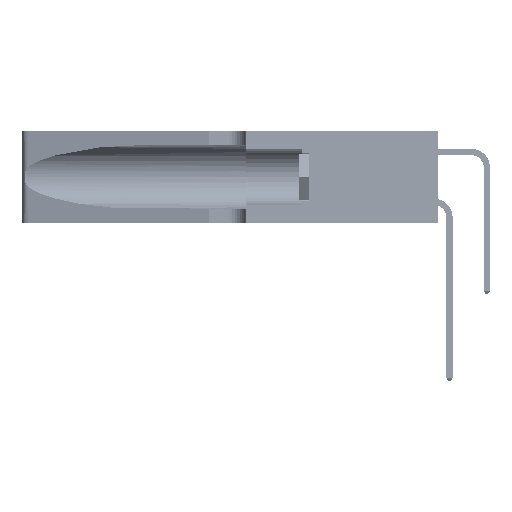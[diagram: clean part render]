
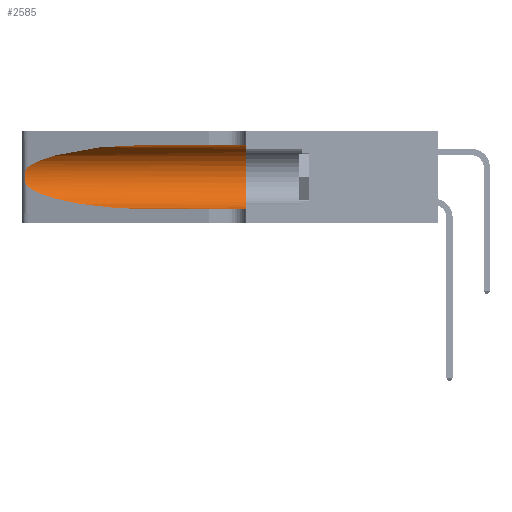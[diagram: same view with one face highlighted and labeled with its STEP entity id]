
A CAD part, left-side view. The second image highlights one B-rep face of the part: STEP entity #2585.
In plain terms, the highlighted cylindrical face has radius 3.308 mm (diameter 6.617 mm), a partial arc.
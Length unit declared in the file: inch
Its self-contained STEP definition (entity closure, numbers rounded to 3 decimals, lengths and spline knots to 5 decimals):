
#133 = LINE ( 'NONE', #42479, #29803 ) ;
#441 = CARTESIAN_POINT ( 'NONE',  ( 0.18966, 0.96281, 0.05475 ) ) ;
#765 = CARTESIAN_POINT ( 'NONE',  ( 0.25789, 1.23486, 0.15765 ) ) ;
#1041 = VERTEX_POINT ( 'NONE', #31571 ) ;
#2025 = VERTEX_POINT ( 'NONE', #5735 ) ;
#2585 = ADVANCED_FACE ( 'NONE', ( #38193 ), #37024, .F. ) ;
#3441 =( BOUNDED_CURVE ( )  B_SPLINE_CURVE ( 3, ( #19033, #22748, #441, #26458 ),
 .UNSPECIFIED., .F., .T. ) 
 B_SPLINE_CURVE_WITH_KNOTS ( ( 4, 4 ),
 ( 3.44316, 4.71239 ),
 .UNSPECIFIED. ) 
 CURVE ( )  GEOMETRIC_REPRESENTATION_ITEM ( )  RATIONAL_B_SPLINE_CURVE ( ( 1., 0.87, 0.87, 1. ) ) 
 REPRESENTATION_ITEM ( '' )  );
#4547 = CARTESIAN_POINT ( 'NONE',  ( 0.25555, 1.22993, 0.14849 ) ) ;
#4876 = ORIENTED_EDGE ( 'NONE', *, *, #35650, .T. ) ;
#5464 = CARTESIAN_POINT ( 'NONE',  ( 0.1305, 0.35, 0.185 ) ) ;
#5735 = CARTESIAN_POINT ( 'NONE',  ( 0.1305, 0.72297, 0.31525 ) ) ;
#5817 = CARTESIAN_POINT ( 'NONE',  ( 0.1305, 0.72297, 0.31525 ) ) ;
#6913 = ORIENTED_EDGE ( 'NONE', *, *, #13393, .F. ) ;
#7002 = CIRCLE ( 'NONE', #17440, 0.13025 ) ;
#8026 = EDGE_CURVE ( 'NONE', #2025, #17849, #10770, .T. ) ;
#8785 = CARTESIAN_POINT ( 'NONE',  ( 0.1305, 1.61858, 0.185 ) ) ;
#9190 = DIRECTION ( 'NONE',  ( 0., 0., 1. ) ) ;
#9556 = CARTESIAN_POINT ( 'NONE',  ( 0.2373, 1.15595, 0.28018 ) ) ;
#9574 = VECTOR ( 'NONE', #47803, 39.37008 ) ;
#10770 = LINE ( 'NONE', #44153, #9574 ) ;
#11849 = CARTESIAN_POINT ( 'NONE',  ( 0.25787, 1.23484, 0.2124 ) ) ;
#13393 = EDGE_CURVE ( 'NONE', #17849, #45125, #7002, .T. ) ;
#15618 = CARTESIAN_POINT ( 'NONE',  ( 0.26018, 1.23835, 0.19895 ) ) ;
#16298 = DIRECTION ( 'NONE',  ( 0., -1., 0. ) ) ;
#16545 = VERTEX_POINT ( 'NONE', #37351 ) ;
#17440 = AXIS2_PLACEMENT_3D ( 'NONE', #5464, #31432, #9190 ) ;
#17849 = VERTEX_POINT ( 'NONE', #35710 ) ;
#19033 = CARTESIAN_POINT ( 'NONE',  ( 0.25487, 1.22718, 0.14631 ) ) ;
#19349 = CARTESIAN_POINT ( 'NONE',  ( 0.26075, 1.23896, 0.178 ) ) ;
#19716 = ORIENTED_EDGE ( 'NONE', *, *, #25425, .T. ) ;
#21882 = ORIENTED_EDGE ( 'NONE', *, *, #47232, .T. ) ;
#22748 = CARTESIAN_POINT ( 'NONE',  ( 0.2373, 1.15595, 0.08982 ) ) ;
#22784 = ORIENTED_EDGE ( 'NONE', *, *, #8026, .F. ) ;
#23077 = CARTESIAN_POINT ( 'NONE',  ( 0.25856, 1.23593, 0.16098 ) ) ;
#25425 = EDGE_CURVE ( 'NONE', #2025, #1041, #29337, .T. ) ;
#25695 = ORIENTED_EDGE ( 'NONE', *, *, #47913, .T. ) ;
#26458 = CARTESIAN_POINT ( 'NONE',  ( 0.1305, 0.72297, 0.05475 ) ) ;
#26766 = CARTESIAN_POINT ( 'NONE',  ( 0.25639, 1.23186, 0.15144 ) ) ;
#28071 = CARTESIAN_POINT ( 'NONE',  ( 0.18966, 0.96281, 0.31525 ) ) ;
#29337 =( BOUNDED_CURVE ( )  B_SPLINE_CURVE ( 3, ( #5817, #28071, #9556, #35576 ),
 .UNSPECIFIED., .F., .F. ) 
 B_SPLINE_CURVE_WITH_KNOTS ( ( 4, 4 ),
 ( 1.5708, 2.84003 ),
 .UNSPECIFIED. ) 
 CURVE ( )  GEOMETRIC_REPRESENTATION_ITEM ( )  RATIONAL_B_SPLINE_CURVE ( ( 1., 0.87, 0.87, 1. ) ) 
 REPRESENTATION_ITEM ( '' )  );
#29803 = VECTOR ( 'NONE', #31468, 39.37008 ) ;
#30338 = CARTESIAN_POINT ( 'NONE',  ( 0.25555, 1.22994, 0.2215 ) ) ;
#30515 = CARTESIAN_POINT ( 'NONE',  ( 0.25487, 1.22718, 0.14631 ) ) ;
#30672 = VERTEX_POINT ( 'NONE', #45387 ) ;
#31014 = DIRECTION ( 'NONE',  ( 0., 0., -1. ) ) ;
#31432 = DIRECTION ( 'NONE',  ( 0., 1., 0. ) ) ;
#31468 = DIRECTION ( 'NONE',  ( 0., -1., 0. ) ) ;
#31571 = CARTESIAN_POINT ( 'NONE',  ( 0.25487, 1.22718, 0.22369 ) ) ;
#32955 = CARTESIAN_POINT ( 'NONE',  ( 0.1305, 0.35, 0.05475 ) ) ;
#34117 = CARTESIAN_POINT ( 'NONE',  ( 0.25639, 1.23184, 0.21858 ) ) ;
#34267 = EDGE_LOOP ( 'NONE', ( #19716, #21882, #4876, #25695, #6913, #22784 ) ) ;
#35576 = CARTESIAN_POINT ( 'NONE',  ( 0.25487, 1.22718, 0.22369 ) ) ;
#35650 = EDGE_CURVE ( 'NONE', #30672, #16545, #3441, .T. ) ;
#35710 = CARTESIAN_POINT ( 'NONE',  ( 0.1305, 0.35, 0.31525 ) ) ;
#37024 = CYLINDRICAL_SURFACE ( 'NONE', #40443, 0.13025 ) ;
#37351 = CARTESIAN_POINT ( 'NONE',  ( 0.1305, 0.72297, 0.05475 ) ) ;
#37853 = CARTESIAN_POINT ( 'NONE',  ( 0.25854, 1.2359, 0.20912 ) ) ;
#38193 = FACE_OUTER_BOUND ( 'NONE', #34267, .T. ) ;
#39461 = B_SPLINE_CURVE_WITH_KNOTS ( 'NONE', 3,
 ( #45053, #30338, #34117, #11849, #37853, #15618, #41547, #19349, #45200, #23077, #765, #26766, #4547, #30515 ),
 .UNSPECIFIED., .F., .F.,
 ( 4, 2, 2, 2, 2, 2, 4 ),
 ( 0., 0.00027, 0.00053, 0.00107, 0.0016, 0.00187, 0.00214 ),
 .UNSPECIFIED. ) ;
#40443 = AXIS2_PLACEMENT_3D ( 'NONE', #8785, #16298, #31014 ) ;
#41547 = CARTESIAN_POINT ( 'NONE',  ( 0.26075, 1.23896, 0.19203 ) ) ;
#42479 = CARTESIAN_POINT ( 'NONE',  ( 0.1305, 1.61858, 0.05475 ) ) ;
#44153 = CARTESIAN_POINT ( 'NONE',  ( 0.1305, 1.61858, 0.31525 ) ) ;
#45053 = CARTESIAN_POINT ( 'NONE',  ( 0.25487, 1.22718, 0.22369 ) ) ;
#45125 = VERTEX_POINT ( 'NONE', #32955 ) ;
#45200 = CARTESIAN_POINT ( 'NONE',  ( 0.26017, 1.23833, 0.17102 ) ) ;
#45387 = CARTESIAN_POINT ( 'NONE',  ( 0.25487, 1.22718, 0.14631 ) ) ;
#47232 = EDGE_CURVE ( 'NONE', #1041, #30672, #39461, .T. ) ;
#47803 = DIRECTION ( 'NONE',  ( 0., -1., 0. ) ) ;
#47913 = EDGE_CURVE ( 'NONE', #16545, #45125, #133, .T. ) ;
